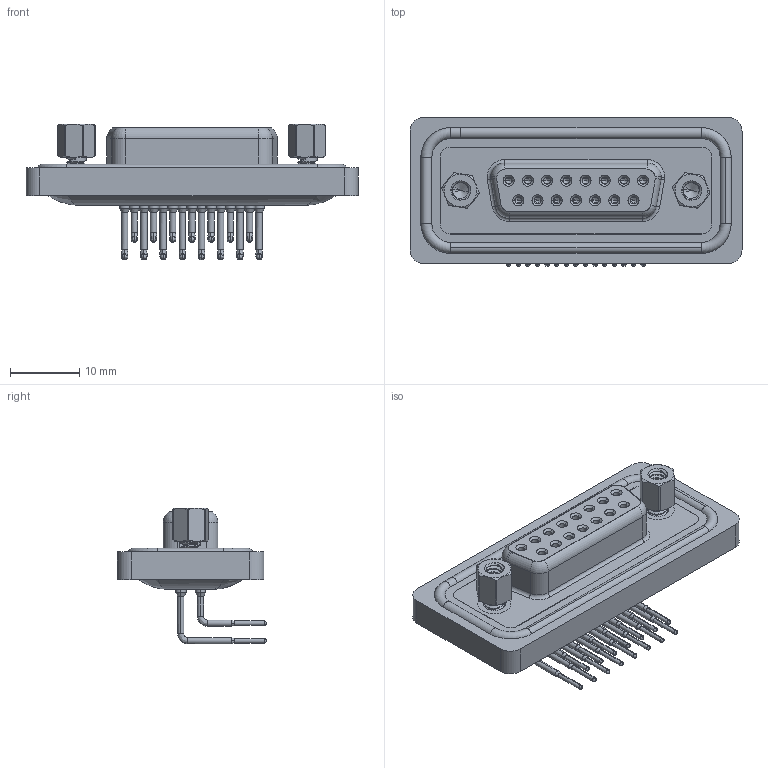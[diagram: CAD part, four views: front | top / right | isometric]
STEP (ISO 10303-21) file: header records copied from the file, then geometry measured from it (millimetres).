
FILE_DESCRIPTION (( 'STEP AP203' ), '1' );
FILE_NAME ('630-W15-640-012.STEP', '2024-04-12T17:31:43', ( '' ), ( '' ), 'SwSTEP 2.0', 'SolidWorks 2023', '' );
FILE_SCHEMA (( 'CONFIG_CONTROL_DESIGN' ));
Length unit declared in the file: millimetre
Products named in the file (8): 630W 4-40 Threaded Rivet_Stabilizer; 630W Contact Row 1; 630W Housing_15 Contacts; 630W Waterproof Housing_15 Contacts; 630-W15-640-012; 630W Contact Row 2; 630W Shell_15 Contacts; 630W 4-40 Hex Standoff
Assembly tree (22 placements, depth 2):
  630-W15-640-012
    630W Housing_15 Contacts
    630W Shell_15 Contacts
    630W Contact Row 1  x8
    630W Contact Row 2  x7
    630W 4-40 Threaded Rivet_Stabilizer  x2
    630W 4-40 Hex Standoff  x2
    630W Waterproof Housing_15 Contacts
Bounding box: 47.89 x 21.5 x 19.59 mm (x, y, z)
Volume: 5547.4 mm3; surface area: 9683 mm2
Topology: 23 solids, 23 shells, 1242 faces, 3179 edges, 2009 vertices
Faces by surface type: cylinder 591, plane 326, cone 193, bspline 82, torus 50
Entity records: 24093 total; most frequent: CARTESIAN_POINT 7743, DIRECTION 3352, ORIENTED_EDGE 3052, EDGE_CURVE 1526, AXIS2_PLACEMENT_3D 1380, VERTEX_POINT 978, EDGE_LOOP 762, CIRCLE 748
